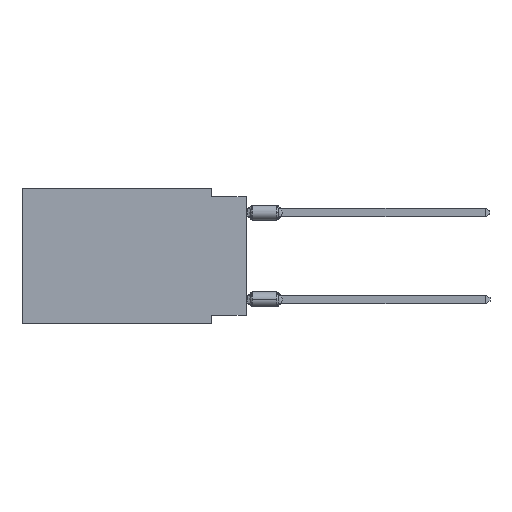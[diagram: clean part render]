
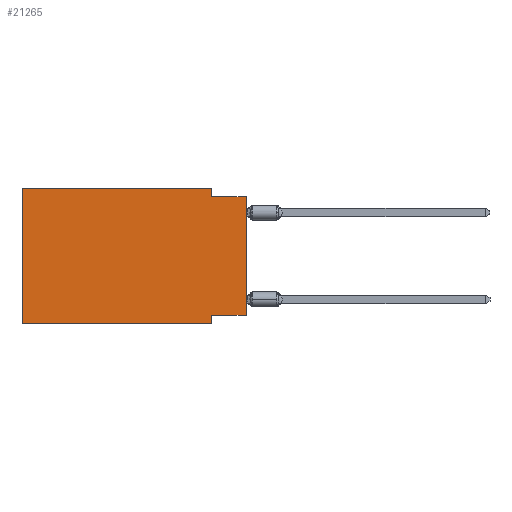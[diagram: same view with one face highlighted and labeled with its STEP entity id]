
A CAD part, left-side view. The second image highlights one B-rep face of the part: STEP entity #21265.
In plain terms, the highlighted planar face has unit normal (-1, 0, 0).
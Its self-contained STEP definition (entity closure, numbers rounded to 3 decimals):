
#729 = CARTESIAN_POINT ( 'NONE',  ( 0., 2.54, -9.906 ) ) ;
#802 = DIRECTION ( 'NONE',  ( 1., 0., 0. ) ) ;
#840 = LINE ( 'NONE', #729, #6743 ) ;
#933 = EDGE_CURVE ( 'NONE', #17393, #14121, #6679, .T. ) ;
#1019 = DIRECTION ( 'NONE',  ( 0., 1., 0. ) ) ;
#1281 = CARTESIAN_POINT ( 'NONE',  ( 0., 2.54, 0. ) ) ;
#2001 = LINE ( 'NONE', #18534, #23148 ) ;
#2003 = CARTESIAN_POINT ( 'NONE',  ( 0., 2.54, -0.635 ) ) ;
#2143 = VERTEX_POINT ( 'NONE', #1281 ) ;
#2843 = ORIENTED_EDGE ( 'NONE', *, *, #21200, .T. ) ;
#3606 = VECTOR ( 'NONE', #1019, 1000. ) ;
#3628 = ORIENTED_EDGE ( 'NONE', *, *, #5902, .F. ) ;
#3994 = CARTESIAN_POINT ( 'NONE',  ( 0., 16.383, -9.906 ) ) ;
#4091 = VECTOR ( 'NONE', #5432, 1000. ) ;
#4122 = LINE ( 'NONE', #3994, #23994 ) ;
#4359 = DIRECTION ( 'NONE',  ( 0., 0., -1. ) ) ;
#4480 = PLANE ( 'NONE',  #9953 ) ;
#4532 = VECTOR ( 'NONE', #19966, 1000. ) ;
#4811 = LINE ( 'NONE', #19382, #3606 ) ;
#5051 = VERTEX_POINT ( 'NONE', #6041 ) ;
#5162 = EDGE_CURVE ( 'NONE', #17393, #23151, #4811, .T. ) ;
#5432 = DIRECTION ( 'NONE',  ( 0., 0., 1. ) ) ;
#5505 = CARTESIAN_POINT ( 'NONE',  ( 0., 2.54, 0. ) ) ;
#5902 = EDGE_CURVE ( 'NONE', #23151, #21127, #840, .T. ) ;
#5996 = DIRECTION ( 'NONE',  ( 0., -1., 0. ) ) ;
#6041 = CARTESIAN_POINT ( 'NONE',  ( 0., 16.383, 0. ) ) ;
#6132 = VECTOR ( 'NONE', #12971, 1000. ) ;
#6679 = LINE ( 'NONE', #20335, #4091 ) ;
#6743 = VECTOR ( 'NONE', #23344, 1000. ) ;
#7239 = CARTESIAN_POINT ( 'NONE',  ( 0., 0., -0.635 ) ) ;
#7391 = DIRECTION ( 'NONE',  ( 0., 0., 1. ) ) ;
#7538 = CARTESIAN_POINT ( 'NONE',  ( 0., 2.54, -9.906 ) ) ;
#7665 = DIRECTION ( 'NONE',  ( 0., -1., 0. ) ) ;
#8384 = CARTESIAN_POINT ( 'NONE',  ( 0., 16.383, 0. ) ) ;
#8662 = ORIENTED_EDGE ( 'NONE', *, *, #16401, .F. ) ;
#9211 = ORIENTED_EDGE ( 'NONE', *, *, #933, .T. ) ;
#9953 = AXIS2_PLACEMENT_3D ( 'NONE', #8384, #802, #4359 ) ;
#11515 = CARTESIAN_POINT ( 'NONE',  ( 0., 0., -0.635 ) ) ;
#11821 = CARTESIAN_POINT ( 'NONE',  ( 0., 0., -9.271 ) ) ;
#12523 = CARTESIAN_POINT ( 'NONE',  ( 0., 16.383, 0. ) ) ;
#12531 = VERTEX_POINT ( 'NONE', #2003 ) ;
#12971 = DIRECTION ( 'NONE',  ( 0., 0., -1. ) ) ;
#14121 = VERTEX_POINT ( 'NONE', #11515 ) ;
#14153 = ORIENTED_EDGE ( 'NONE', *, *, #5162, .F. ) ;
#14342 = ORIENTED_EDGE ( 'NONE', *, *, #15211, .F. ) ;
#14354 = VERTEX_POINT ( 'NONE', #18243 ) ;
#15211 = EDGE_CURVE ( 'NONE', #12531, #14121, #23976, .T. ) ;
#15598 = EDGE_CURVE ( 'NONE', #2143, #12531, #22244, .T. ) ;
#16322 = ORIENTED_EDGE ( 'NONE', *, *, #15598, .F. ) ;
#16401 = EDGE_CURVE ( 'NONE', #14354, #5051, #2001, .T. ) ;
#17131 = EDGE_LOOP ( 'NONE', ( #9211, #14342, #16322, #21105, #8662, #2843, #3628, #14153 ) ) ;
#17393 = VERTEX_POINT ( 'NONE', #11821 ) ;
#17817 = FACE_OUTER_BOUND ( 'NONE', #17131, .T. ) ;
#18243 = CARTESIAN_POINT ( 'NONE',  ( 0., 16.383, -9.906 ) ) ;
#18534 = CARTESIAN_POINT ( 'NONE',  ( 0., 16.383, 0. ) ) ;
#19382 = CARTESIAN_POINT ( 'NONE',  ( 0., 0., -9.271 ) ) ;
#19966 = DIRECTION ( 'NONE',  ( 0., -1., 0. ) ) ;
#20335 = CARTESIAN_POINT ( 'NONE',  ( 0., 0., 0. ) ) ;
#20882 = CARTESIAN_POINT ( 'NONE',  ( 0., 2.54, -9.271 ) ) ;
#21105 = ORIENTED_EDGE ( 'NONE', *, *, #21780, .F. ) ;
#21127 = VERTEX_POINT ( 'NONE', #7538 ) ;
#21200 = EDGE_CURVE ( 'NONE', #14354, #21127, #4122, .T. ) ;
#21265 = ADVANCED_FACE ( 'NONE', ( #17817 ), #4480, .F. ) ;
#21328 = VECTOR ( 'NONE', #5996, 1000. ) ;
#21780 = EDGE_CURVE ( 'NONE', #5051, #2143, #23612, .T. ) ;
#22244 = LINE ( 'NONE', #5505, #6132 ) ;
#23148 = VECTOR ( 'NONE', #7391, 1000. ) ;
#23151 = VERTEX_POINT ( 'NONE', #20882 ) ;
#23344 = DIRECTION ( 'NONE',  ( 0., 0., -1. ) ) ;
#23612 = LINE ( 'NONE', #12523, #4532 ) ;
#23976 = LINE ( 'NONE', #7239, #21328 ) ;
#23994 = VECTOR ( 'NONE', #7665, 1000. ) ;
